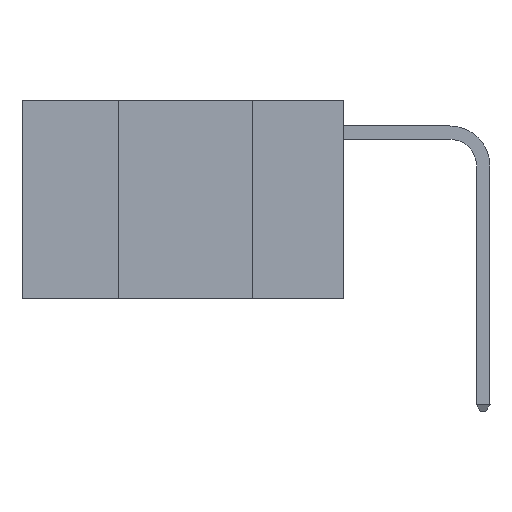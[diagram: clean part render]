
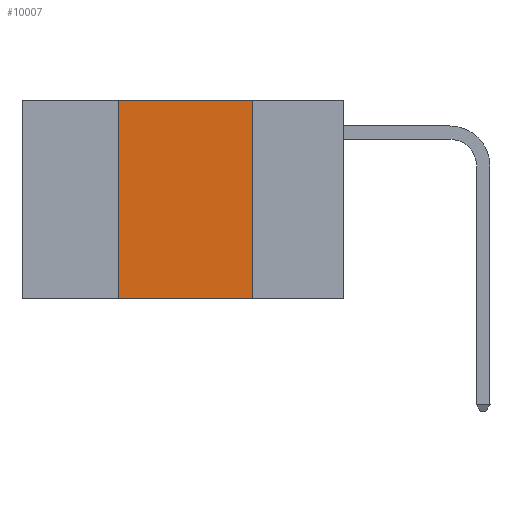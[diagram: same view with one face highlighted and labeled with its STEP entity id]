
A CAD part, left-side view. The second image highlights one B-rep face of the part: STEP entity #10007.
In plain terms, the highlighted planar face has unit normal (-1, 0, 0).
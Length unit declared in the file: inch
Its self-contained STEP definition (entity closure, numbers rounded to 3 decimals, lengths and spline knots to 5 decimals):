
#64 = CARTESIAN_POINT ( 'NONE',  ( 0., 0.17, 0. ) ) ;
#1153 = VECTOR ( 'NONE', #15569, 39.37008 ) ;
#1242 = VERTEX_POINT ( 'NONE', #11740 ) ;
#1342 = DIRECTION ( 'NONE',  ( 0., 0., 1. ) ) ;
#2028 = VECTOR ( 'NONE', #15952, 39.37008 ) ;
#2332 = ORIENTED_EDGE ( 'NONE', *, *, #14774, .F. ) ;
#2404 = LINE ( 'NONE', #11770, #6584 ) ;
#4855 = DIRECTION ( 'NONE',  ( 0., -1., 0. ) ) ;
#4946 = LINE ( 'NONE', #14198, #1153 ) ;
#5475 = EDGE_LOOP ( 'NONE', ( #13761, #6943, #2332, #14095 ) ) ;
#6019 = VERTEX_POINT ( 'NONE', #64 ) ;
#6584 = VECTOR ( 'NONE', #4855, 39.37008 ) ;
#6690 = DIRECTION ( 'NONE',  ( 1., 0., 0. ) ) ;
#6943 = ORIENTED_EDGE ( 'NONE', *, *, #17374, .F. ) ;
#7779 = CARTESIAN_POINT ( 'NONE',  ( 0., 0.42, 0. ) ) ;
#9361 = FACE_OUTER_BOUND ( 'NONE', #5475, .T. ) ;
#9751 = CARTESIAN_POINT ( 'NONE',  ( 0., 0.42, 0. ) ) ;
#9908 = LINE ( 'NONE', #14607, #2028 ) ;
#9950 = AXIS2_PLACEMENT_3D ( 'NONE', #14933, #6690, #16281 ) ;
#9979 = CARTESIAN_POINT ( 'NONE',  ( 0., 0.17, -0.37 ) ) ;
#10007 = ADVANCED_FACE ( 'NONE', ( #9361 ), #10811, .F. ) ;
#10811 = PLANE ( 'NONE',  #9950 ) ;
#11740 = CARTESIAN_POINT ( 'NONE',  ( 0., 0.42, -0.37 ) ) ;
#11747 = VECTOR ( 'NONE', #1342, 39.37008 ) ;
#11770 = CARTESIAN_POINT ( 'NONE',  ( 0., 0.6, -0.37 ) ) ;
#13761 = ORIENTED_EDGE ( 'NONE', *, *, #16569, .F. ) ;
#13831 = EDGE_CURVE ( 'NONE', #1242, #17802, #2404, .T. ) ;
#14095 = ORIENTED_EDGE ( 'NONE', *, *, #13831, .T. ) ;
#14198 = CARTESIAN_POINT ( 'NONE',  ( 0., 0.17, 0. ) ) ;
#14607 = CARTESIAN_POINT ( 'NONE',  ( 0., 0.6, 0. ) ) ;
#14774 = EDGE_CURVE ( 'NONE', #1242, #17395, #14937, .T. ) ;
#14933 = CARTESIAN_POINT ( 'NONE',  ( 0., 0.6, 0. ) ) ;
#14937 = LINE ( 'NONE', #9751, #11747 ) ;
#15569 = DIRECTION ( 'NONE',  ( 0., 0., -1. ) ) ;
#15952 = DIRECTION ( 'NONE',  ( 0., -1., 0. ) ) ;
#16281 = DIRECTION ( 'NONE',  ( 0., 0., -1. ) ) ;
#16569 = EDGE_CURVE ( 'NONE', #6019, #17802, #4946, .T. ) ;
#17374 = EDGE_CURVE ( 'NONE', #17395, #6019, #9908, .T. ) ;
#17395 = VERTEX_POINT ( 'NONE', #7779 ) ;
#17802 = VERTEX_POINT ( 'NONE', #9979 ) ;
